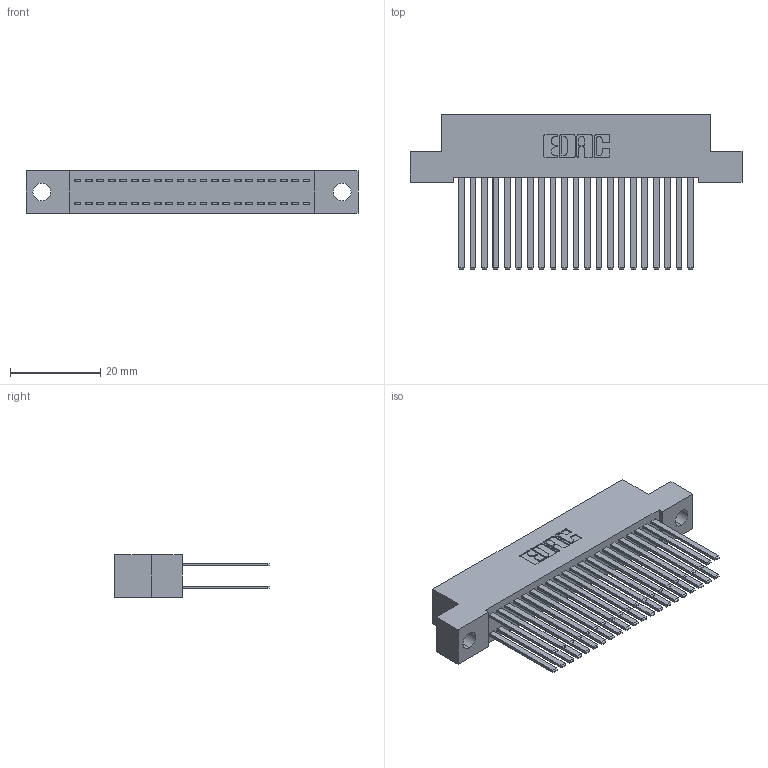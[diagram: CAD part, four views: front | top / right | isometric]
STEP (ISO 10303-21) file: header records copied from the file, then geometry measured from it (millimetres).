
FILE_DESCRIPTION (( 'STEP AP203' ), '1' );
FILE_NAME ('392-042-544-204.STEP', '2018-08-16T13:50:36', ( '' ), ( '' ), 'SwSTEP 2.0', 'SolidWorks 2016', '' );
FILE_SCHEMA (( 'CONFIG_CONTROL_DESIGN' ));
Length unit declared in the file: inch
Products named in the file (3): 342 Part_.156 TH; 345-292-001_345-293-144; 392-042-544-204
Assembly tree (43 placements, depth 2):
  392-042-544-204
    342 Part_.156 TH
    345-292-001_345-293-144  x42
Bounding box: 73.66 x 34.3 x 9.4 mm (x, y, z)
Volume: 7020.7 mm3; surface area: 12365.1 mm2
Topology: 43 solids, 43 shells, 2042 faces, 6053 edges, 3978 vertices
Faces by surface type: plane 1410, cylinder 632
Entity records: 15913 total; most frequent: CARTESIAN_POINT 2658, ORIENTED_EDGE 2594, DIRECTION 2305, EDGE_CURVE 1297, LINE 1173, VECTOR 1173, VERTEX_POINT 862, AXIS2_PLACEMENT_3D 566
